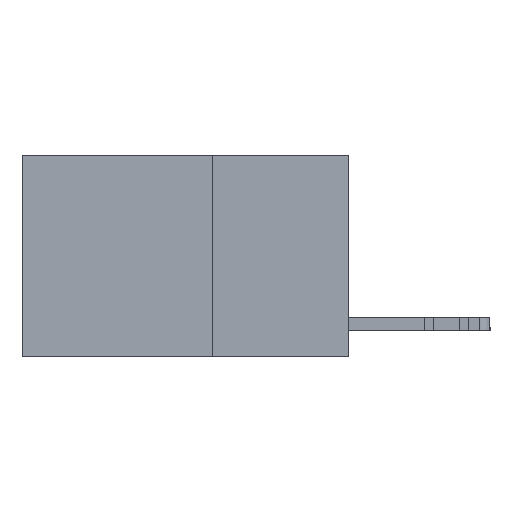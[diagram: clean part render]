
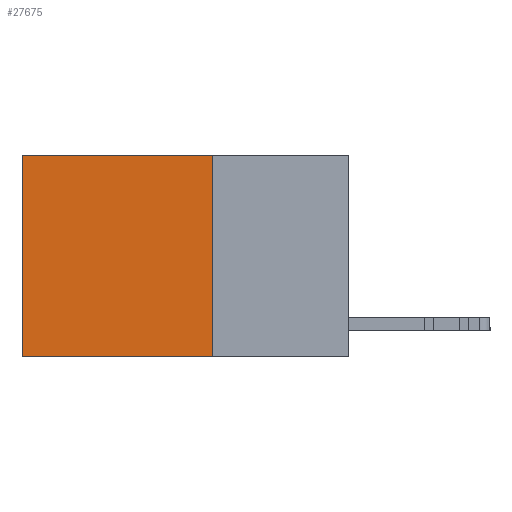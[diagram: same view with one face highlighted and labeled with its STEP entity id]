
A CAD part, left-side view. The second image highlights one B-rep face of the part: STEP entity #27675.
In plain terms, the highlighted planar face has unit normal (-1, 0, 0).
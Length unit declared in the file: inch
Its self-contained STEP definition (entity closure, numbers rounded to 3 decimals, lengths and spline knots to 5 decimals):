
#311 = VECTOR ( 'NONE', #20520, 39.37008 ) ;
#436 = AXIS2_PLACEMENT_3D ( 'NONE', #6162, #10717, #29877 ) ;
#1317 = EDGE_CURVE ( 'NONE', #18325, #2899, #15728, .T. ) ;
#1803 = ORIENTED_EDGE ( 'NONE', *, *, #19398, .F. ) ;
#2029 = EDGE_CURVE ( 'NONE', #28965, #18325, #11370, .T. ) ;
#2259 = CARTESIAN_POINT ( 'NONE',  ( 0.2625, 0.6, 0. ) ) ;
#2899 = VERTEX_POINT ( 'NONE', #6747 ) ;
#3494 = VERTEX_POINT ( 'NONE', #30453 ) ;
#3823 = CARTESIAN_POINT ( 'NONE',  ( 0.2625, 0.6, 0. ) ) ;
#5857 = FACE_OUTER_BOUND ( 'NONE', #9085, .T. ) ;
#6162 = CARTESIAN_POINT ( 'NONE',  ( 0.2625, 0.25, 0. ) ) ;
#6402 = VECTOR ( 'NONE', #17245, 39.37008 ) ;
#6747 = CARTESIAN_POINT ( 'NONE',  ( 0.2625, 0.6, -0.37 ) ) ;
#9085 = EDGE_LOOP ( 'NONE', ( #27022, #1803, #29711, #11926 ) ) ;
#9492 = LINE ( 'NONE', #23616, #311 ) ;
#10717 = DIRECTION ( 'NONE',  ( 1., 0., 0. ) ) ;
#11061 = VECTOR ( 'NONE', #27134, 39.37008 ) ;
#11370 = LINE ( 'NONE', #24765, #11061 ) ;
#11926 = ORIENTED_EDGE ( 'NONE', *, *, #2029, .T. ) ;
#15271 = DIRECTION ( 'NONE',  ( 0., 0., -1. ) ) ;
#15728 = LINE ( 'NONE', #3823, #16023 ) ;
#16023 = VECTOR ( 'NONE', #15271, 39.37008 ) ;
#16413 = CARTESIAN_POINT ( 'NONE',  ( 0.2625, 0.25, 0. ) ) ;
#17245 = DIRECTION ( 'NONE',  ( 0., 1., 0. ) ) ;
#18307 = EDGE_CURVE ( 'NONE', #28965, #3494, #9492, .T. ) ;
#18325 = VERTEX_POINT ( 'NONE', #2259 ) ;
#19121 = LINE ( 'NONE', #21340, #6402 ) ;
#19398 = EDGE_CURVE ( 'NONE', #3494, #2899, #19121, .T. ) ;
#20520 = DIRECTION ( 'NONE',  ( 0., 0., -1. ) ) ;
#21340 = CARTESIAN_POINT ( 'NONE',  ( 0.2625, 0.25, -0.37 ) ) ;
#22782 = PLANE ( 'NONE',  #436 ) ;
#23616 = CARTESIAN_POINT ( 'NONE',  ( 0.2625, 0.25, 0. ) ) ;
#24765 = CARTESIAN_POINT ( 'NONE',  ( 0.2625, 0.25, 0. ) ) ;
#27022 = ORIENTED_EDGE ( 'NONE', *, *, #1317, .T. ) ;
#27134 = DIRECTION ( 'NONE',  ( 0., 1., 0. ) ) ;
#27675 = ADVANCED_FACE ( 'NONE', ( #5857 ), #22782, .F. ) ;
#28965 = VERTEX_POINT ( 'NONE', #16413 ) ;
#29711 = ORIENTED_EDGE ( 'NONE', *, *, #18307, .F. ) ;
#29877 = DIRECTION ( 'NONE',  ( 0., 0., -1. ) ) ;
#30453 = CARTESIAN_POINT ( 'NONE',  ( 0.2625, 0.25, -0.37 ) ) ;
